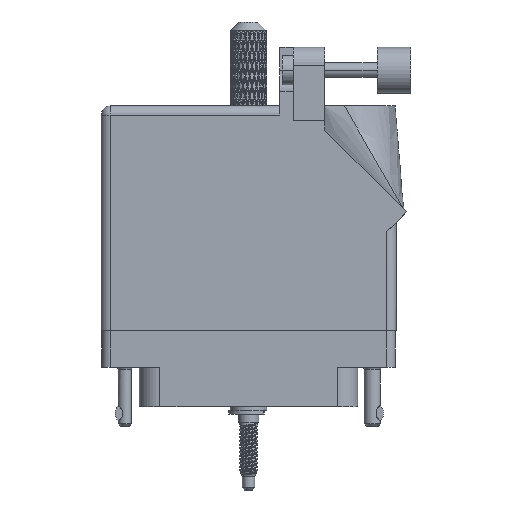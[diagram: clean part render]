
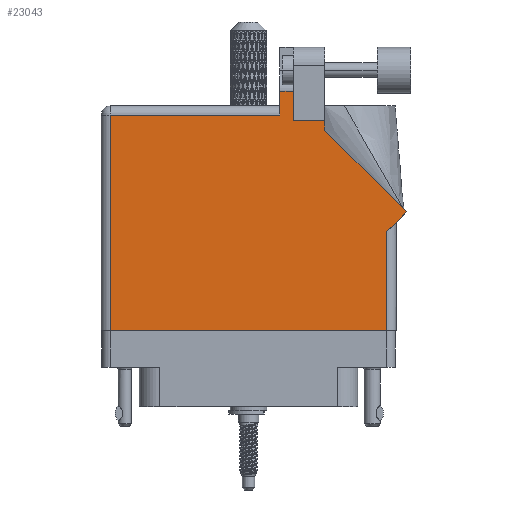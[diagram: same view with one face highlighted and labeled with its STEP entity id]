
A CAD part, front view. The second image highlights one B-rep face of the part: STEP entity #23043.
In plain terms, the highlighted face is planar.
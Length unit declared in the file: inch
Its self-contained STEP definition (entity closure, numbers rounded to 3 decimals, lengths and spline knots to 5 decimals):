
#945 = ORIENTED_EDGE ( 'NONE', *, *, #61962, .T. ) ;
#1937 = DIRECTION ( 'NONE',  ( 0.707, 0.707, 0. ) ) ;
#5305 = ORIENTED_EDGE ( 'NONE', *, *, #22033, .T. ) ;
#9261 = VERTEX_POINT ( 'NONE', #69567 ) ;
#11638 = CARTESIAN_POINT ( 'NONE',  ( -0.943, -0.1, 0.455 ) ) ;
#11849 = ORIENTED_EDGE ( 'NONE', *, *, #12734, .T. ) ;
#12721 = VERTEX_POINT ( 'NONE', #20640 ) ;
#12734 = EDGE_CURVE ( 'NONE', #94383, #73897, #20009, .T. ) ;
#14743 = LINE ( 'NONE', #80844, #80194 ) ;
#15353 = DIRECTION ( 'NONE',  ( -1., 0., 0. ) ) ;
#17224 = VECTOR ( 'NONE', #75474, 39.37008 ) ;
#17386 = PLANE ( 'NONE',  #29991 ) ;
#18976 = DIRECTION ( 'NONE',  ( -1., 0., 0. ) ) ;
#20009 = LINE ( 'NONE', #92582, #17224 ) ;
#20583 = CARTESIAN_POINT ( 'NONE',  ( -1.005, -0.1, 0.455 ) ) ;
#20640 = CARTESIAN_POINT ( 'NONE',  ( 1.07571, 0.70771, 0.455 ) ) ;
#21346 = LINE ( 'NONE', #92000, #22785 ) ;
#22033 = EDGE_CURVE ( 'NONE', #100439, #70642, #75394, .T. ) ;
#22785 = VECTOR ( 'NONE', #38742, 39.37008 ) ;
#23043 = ADVANCED_FACE ( 'NONE', ( #25165 ), #17386, .F. ) ;
#24977 = ORIENTED_EDGE ( 'NONE', *, *, #26974, .T. ) ;
#25016 = EDGE_LOOP ( 'NONE', ( #29225, #47947, #11849, #24977, #32954, #77447, #5305, #113136, #48288, #97106, #945 ) ) ;
#25165 = FACE_OUTER_BOUND ( 'NONE', #25016, .T. ) ;
#26974 = EDGE_CURVE ( 'NONE', #73897, #97032, #63614, .T. ) ;
#27023 = VERTEX_POINT ( 'NONE', #64118 ) ;
#29225 = ORIENTED_EDGE ( 'NONE', *, *, #29504, .T. ) ;
#29504 = EDGE_CURVE ( 'NONE', #9261, #40960, #21346, .T. ) ;
#29687 = CARTESIAN_POINT ( 'NONE',  ( 1.07571, 0.70771, 0.455 ) ) ;
#29991 = AXIS2_PLACEMENT_3D ( 'NONE', #71410, #79600, #35247 ) ;
#32954 = ORIENTED_EDGE ( 'NONE', *, *, #87877, .T. ) ;
#34627 = LINE ( 'NONE', #87353, #36086 ) ;
#35247 = DIRECTION ( 'NONE',  ( -1., 0., 0. ) ) ;
#36086 = VECTOR ( 'NONE', #15353, 39.37008 ) ;
#36867 = EDGE_CURVE ( 'NONE', #12721, #27023, #51144, .T. ) ;
#38742 = DIRECTION ( 'NONE',  ( 0., 1., 0. ) ) ;
#39589 = CARTESIAN_POINT ( 'NONE',  ( 0.212, 1.368, 0.455 ) ) ;
#40960 = VERTEX_POINT ( 'NONE', #77318 ) ;
#43122 = CARTESIAN_POINT ( 'NONE',  ( 0.519, 1.26442, 0.455 ) ) ;
#45249 = EDGE_CURVE ( 'NONE', #70642, #12721, #67113, .T. ) ;
#47433 = VECTOR ( 'NONE', #81657, 39.37008 ) ;
#47947 = ORIENTED_EDGE ( 'NONE', *, *, #101933, .T. ) ;
#48288 = ORIENTED_EDGE ( 'NONE', *, *, #36867, .T. ) ;
#51144 = LINE ( 'NONE', #29687, #112318 ) ;
#53071 = CARTESIAN_POINT ( 'NONE',  ( 0.943, 0.575, 0.455 ) ) ;
#53445 = DIRECTION ( 'NONE',  ( 0., -1., 0. ) ) ;
#54949 = CARTESIAN_POINT ( 'NONE',  ( 1.005, 0.637, 0.455 ) ) ;
#54965 = CARTESIAN_POINT ( 'NONE',  ( -0.943, -0.1, 0.455 ) ) ;
#55879 = DIRECTION ( 'NONE',  ( -0.707, 0.707, 0. ) ) ;
#57607 = CARTESIAN_POINT ( 'NONE',  ( 0.212, 1.5315, 0.455 ) ) ;
#58879 = EDGE_CURVE ( 'NONE', #103074, #100439, #110102, .T. ) ;
#61962 = EDGE_CURVE ( 'NONE', #98420, #9261, #34627, .T. ) ;
#62174 = LINE ( 'NONE', #54965, #64951 ) ;
#62613 = DIRECTION ( 'NONE',  ( -1., 0., 0. ) ) ;
#63614 = LINE ( 'NONE', #72259, #95587 ) ;
#64118 = CARTESIAN_POINT ( 'NONE',  ( 0.519, 1.26442, 0.455 ) ) ;
#64951 = VECTOR ( 'NONE', #53445, 39.37008 ) ;
#67113 = LINE ( 'NONE', #54949, #79598 ) ;
#69179 = DIRECTION ( 'NONE',  ( 0., 1., 0. ) ) ;
#69567 = CARTESIAN_POINT ( 'NONE',  ( 0.306, 1.33, 0.455 ) ) ;
#70183 = CARTESIAN_POINT ( 'NONE',  ( 0.943, 0.637, 0.455 ) ) ;
#70642 = VERTEX_POINT ( 'NONE', #53071 ) ;
#71410 = CARTESIAN_POINT ( 'NONE',  ( -1.005, 1.43, 0.455 ) ) ;
#72259 = CARTESIAN_POINT ( 'NONE',  ( -1.005, 1.368, 0.455 ) ) ;
#73897 = VERTEX_POINT ( 'NONE', #39589 ) ;
#75394 = LINE ( 'NONE', #70183, #83756 ) ;
#75474 = DIRECTION ( 'NONE',  ( 0., -1., 0. ) ) ;
#77318 = CARTESIAN_POINT ( 'NONE',  ( 0.306, 1.5315, 0.455 ) ) ;
#77447 = ORIENTED_EDGE ( 'NONE', *, *, #58879, .T. ) ;
#79119 = EDGE_CURVE ( 'NONE', #27023, #98420, #96750, .T. ) ;
#79598 = VECTOR ( 'NONE', #1937, 39.37008 ) ;
#79600 = DIRECTION ( 'NONE',  ( 0., 0., -1. ) ) ;
#80194 = VECTOR ( 'NONE', #62613, 39.37008 ) ;
#80844 = CARTESIAN_POINT ( 'NONE',  ( 0.63677, 1.5315, 0.455 ) ) ;
#81657 = DIRECTION ( 'NONE',  ( 1., 0., 0. ) ) ;
#83756 = VECTOR ( 'NONE', #114465, 39.37008 ) ;
#87353 = CARTESIAN_POINT ( 'NONE',  ( 0.519, 1.33, 0.455 ) ) ;
#87877 = EDGE_CURVE ( 'NONE', #97032, #103074, #62174, .T. ) ;
#89076 = CARTESIAN_POINT ( 'NONE',  ( -0.943, 1.368, 0.455 ) ) ;
#92000 = CARTESIAN_POINT ( 'NONE',  ( 0.306, 1.33, 0.455 ) ) ;
#92582 = CARTESIAN_POINT ( 'NONE',  ( 0.212, 1.43, 0.455 ) ) ;
#93775 = CARTESIAN_POINT ( 'NONE',  ( 0.943, -0.1, 0.455 ) ) ;
#94383 = VERTEX_POINT ( 'NONE', #57607 ) ;
#95381 = VECTOR ( 'NONE', #69179, 39.37008 ) ;
#95587 = VECTOR ( 'NONE', #18976, 39.37008 ) ;
#96750 = LINE ( 'NONE', #43122, #95381 ) ;
#97032 = VERTEX_POINT ( 'NONE', #89076 ) ;
#97106 = ORIENTED_EDGE ( 'NONE', *, *, #79119, .T. ) ;
#98420 = VERTEX_POINT ( 'NONE', #100413 ) ;
#100413 = CARTESIAN_POINT ( 'NONE',  ( 0.519, 1.33, 0.455 ) ) ;
#100439 = VERTEX_POINT ( 'NONE', #93775 ) ;
#101933 = EDGE_CURVE ( 'NONE', #40960, #94383, #14743, .T. ) ;
#103074 = VERTEX_POINT ( 'NONE', #11638 ) ;
#110102 = LINE ( 'NONE', #20583, #47433 ) ;
#112318 = VECTOR ( 'NONE', #55879, 39.37008 ) ;
#113136 = ORIENTED_EDGE ( 'NONE', *, *, #45249, .T. ) ;
#114465 = DIRECTION ( 'NONE',  ( 0., 1., 0. ) ) ;
